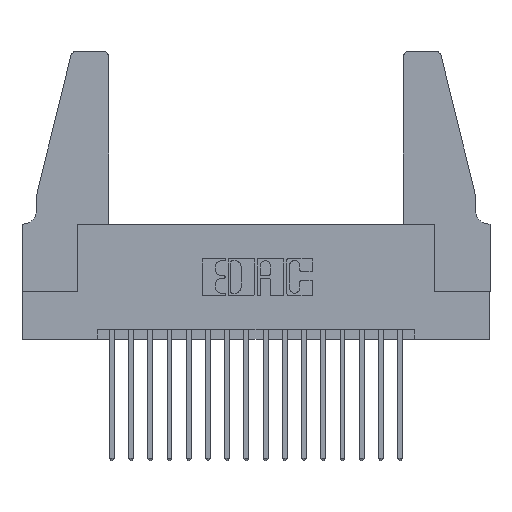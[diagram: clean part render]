
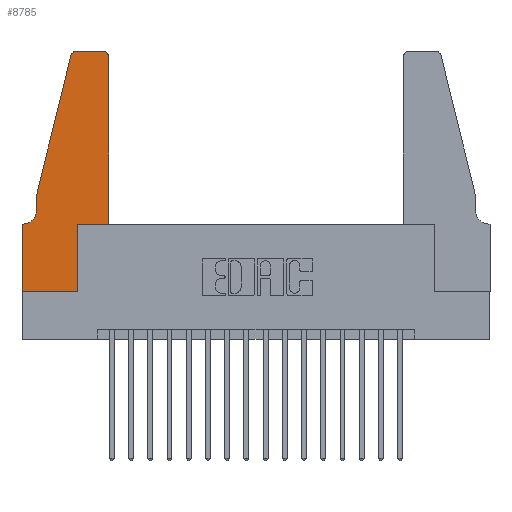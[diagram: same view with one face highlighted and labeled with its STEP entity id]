
A CAD part, top view. The second image highlights one B-rep face of the part: STEP entity #8785.
In plain terms, the highlighted planar face has unit normal (0, 0, 1).
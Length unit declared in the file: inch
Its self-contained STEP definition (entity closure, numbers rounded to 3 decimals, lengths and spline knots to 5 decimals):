
#44 = EDGE_CURVE ( 'NONE', #2629, #17191, #13344, .T. ) ;
#200 = ORIENTED_EDGE ( 'NONE', *, *, #10529, .T. ) ;
#275 = CARTESIAN_POINT ( 'NONE',  ( 0., 0., 0.37 ) ) ;
#299 = CIRCLE ( 'NONE', #2909, 0.03 ) ;
#307 = DIRECTION ( 'NONE',  ( 0., 0., 1. ) ) ;
#358 = CARTESIAN_POINT ( 'NONE',  ( 0.0755, 0.35, 0.37 ) ) ;
#796 = LINE ( 'NONE', #5725, #4197 ) ;
#1112 = VECTOR ( 'NONE', #12012, 39.37008 ) ;
#1293 = VERTEX_POINT ( 'NONE', #12576 ) ;
#1413 = ORIENTED_EDGE ( 'NONE', *, *, #2693, .T. ) ;
#1495 = ORIENTED_EDGE ( 'NONE', *, *, #4208, .T. ) ;
#1847 = EDGE_CURVE ( 'NONE', #10890, #1293, #4965, .T. ) ;
#2177 = CARTESIAN_POINT ( 'NONE',  ( 0., 0., 0.37 ) ) ;
#2473 = LINE ( 'NONE', #5337, #14990 ) ;
#2553 = ORIENTED_EDGE ( 'NONE', *, *, #11028, .T. ) ;
#2623 = EDGE_CURVE ( 'NONE', #10138, #3721, #7997, .T. ) ;
#2629 = VERTEX_POINT ( 'NONE', #18126 ) ;
#2693 = EDGE_CURVE ( 'NONE', #9091, #14931, #2473, .T. ) ;
#2798 = CIRCLE ( 'NONE', #15040, 0.03 ) ;
#2909 = AXIS2_PLACEMENT_3D ( 'NONE', #16535, #8166, #17917 ) ;
#3327 = DIRECTION ( 'NONE',  ( 0., 1., 0. ) ) ;
#3484 = CARTESIAN_POINT ( 'NONE',  ( 0.25487, 1.22718, 0.37 ) ) ;
#3504 = DIRECTION ( 'NONE',  ( -1., 0., 0. ) ) ;
#3545 = DIRECTION ( 'NONE',  ( -0.239, -0.971, 0. ) ) ;
#3574 = CARTESIAN_POINT ( 'NONE',  ( 0.2865, 0., 0.37 ) ) ;
#3633 = CARTESIAN_POINT ( 'NONE',  ( 0.2865, 0.35, 0.37 ) ) ;
#3721 = VERTEX_POINT ( 'NONE', #17758 ) ;
#4163 = CIRCLE ( 'NONE', #10090, 0.07 ) ;
#4197 = VECTOR ( 'NONE', #16907, 39.37008 ) ;
#4208 = EDGE_CURVE ( 'NONE', #12950, #10890, #7707, .T. ) ;
#4421 = EDGE_CURVE ( 'NONE', #15932, #12950, #12097, .T. ) ;
#4439 = AXIS2_PLACEMENT_3D ( 'NONE', #5583, #16766, #8406 ) ;
#4965 = LINE ( 'NONE', #11973, #1112 ) ;
#5068 = CARTESIAN_POINT ( 'NONE',  ( 0.0755, 0.5, 0.37 ) ) ;
#5165 = CARTESIAN_POINT ( 'NONE',  ( 0.0055, 0.42, 0.37 ) ) ;
#5242 = ORIENTED_EDGE ( 'NONE', *, *, #15575, .T. ) ;
#5337 = CARTESIAN_POINT ( 'NONE',  ( 0.0755, 0.5, 0.37 ) ) ;
#5452 = CARTESIAN_POINT ( 'NONE',  ( 0.2605, 1.25, 0.37 ) ) ;
#5583 = CARTESIAN_POINT ( 'NONE',  ( 0., 0.35, 0.37 ) ) ;
#5725 = CARTESIAN_POINT ( 'NONE',  ( 0.0755, 0.5, 0.37 ) ) ;
#6577 = DIRECTION ( 'NONE',  ( -1., 0., 0. ) ) ;
#6728 = LINE ( 'NONE', #8404, #17420 ) ;
#6967 = EDGE_CURVE ( 'NONE', #1293, #12687, #6728, .T. ) ;
#7138 = CARTESIAN_POINT ( 'NONE',  ( 0.4505, 1.22, 0.37 ) ) ;
#7577 = CARTESIAN_POINT ( 'NONE',  ( 0.4205, 1.25, 0.37 ) ) ;
#7707 = LINE ( 'NONE', #13160, #11421 ) ;
#7997 = LINE ( 'NONE', #5452, #14553 ) ;
#8166 = DIRECTION ( 'NONE',  ( 0., 0., 1. ) ) ;
#8404 = CARTESIAN_POINT ( 'NONE',  ( 0.4505, 0.35, 0.37 ) ) ;
#8406 = DIRECTION ( 'NONE',  ( 1., 0., 0. ) ) ;
#8519 = CARTESIAN_POINT ( 'NONE',  ( 0., 0., 0.37 ) ) ;
#8765 = EDGE_LOOP ( 'NONE', ( #14746, #9047, #1413, #200, #13914, #10304, #5242, #17519, #1495, #16688, #12825, #2553 ) ) ;
#8785 = ADVANCED_FACE ( 'NONE', ( #15851 ), #11148, .T. ) ;
#8878 = CARTESIAN_POINT ( 'NONE',  ( 0.284, 1.22, 0.37 ) ) ;
#9047 = ORIENTED_EDGE ( 'NONE', *, *, #14766, .T. ) ;
#9091 = VERTEX_POINT ( 'NONE', #3484 ) ;
#9843 = DIRECTION ( 'NONE',  ( -1., 0., 0. ) ) ;
#10039 = VECTOR ( 'NONE', #3504, 39.37008 ) ;
#10090 = AXIS2_PLACEMENT_3D ( 'NONE', #5165, #14939, #6577 ) ;
#10138 = VERTEX_POINT ( 'NONE', #7577 ) ;
#10254 = DIRECTION ( 'NONE',  ( 1., 0., 0. ) ) ;
#10304 = ORIENTED_EDGE ( 'NONE', *, *, #44, .T. ) ;
#10529 = EDGE_CURVE ( 'NONE', #14931, #17115, #796, .T. ) ;
#10890 = VERTEX_POINT ( 'NONE', #3633 ) ;
#10913 = VECTOR ( 'NONE', #15836, 39.37008 ) ;
#11028 = EDGE_CURVE ( 'NONE', #12687, #10138, #299, .T. ) ;
#11148 = PLANE ( 'NONE',  #4439 ) ;
#11421 = VECTOR ( 'NONE', #3327, 39.37008 ) ;
#11483 = EDGE_CURVE ( 'NONE', #17115, #2629, #4163, .T. ) ;
#11973 = CARTESIAN_POINT ( 'NONE',  ( 0.4505, 0.35, 0.37 ) ) ;
#12012 = DIRECTION ( 'NONE',  ( 1., 0., 0. ) ) ;
#12097 = LINE ( 'NONE', #2177, #15350 ) ;
#12100 = DIRECTION ( 'NONE',  ( 1., 0., 0. ) ) ;
#12576 = CARTESIAN_POINT ( 'NONE',  ( 0.4505, 0.35, 0.37 ) ) ;
#12687 = VERTEX_POINT ( 'NONE', #7138 ) ;
#12825 = ORIENTED_EDGE ( 'NONE', *, *, #6967, .T. ) ;
#12950 = VERTEX_POINT ( 'NONE', #3574 ) ;
#13160 = CARTESIAN_POINT ( 'NONE',  ( 0.2865, 0.35, 0.37 ) ) ;
#13344 = LINE ( 'NONE', #358, #10039 ) ;
#13682 = CARTESIAN_POINT ( 'NONE',  ( 0.0755, 0.42, 0.37 ) ) ;
#13914 = ORIENTED_EDGE ( 'NONE', *, *, #11483, .T. ) ;
#14553 = VECTOR ( 'NONE', #9843, 39.37008 ) ;
#14642 = LINE ( 'NONE', #275, #10913 ) ;
#14746 = ORIENTED_EDGE ( 'NONE', *, *, #2623, .T. ) ;
#14766 = EDGE_CURVE ( 'NONE', #3721, #9091, #2798, .T. ) ;
#14931 = VERTEX_POINT ( 'NONE', #5068 ) ;
#14939 = DIRECTION ( 'NONE',  ( 0., 0., -1. ) ) ;
#14990 = VECTOR ( 'NONE', #3545, 39.37008 ) ;
#15040 = AXIS2_PLACEMENT_3D ( 'NONE', #8878, #307, #10254 ) ;
#15240 = CARTESIAN_POINT ( 'NONE',  ( 0., 0.35, 0.37 ) ) ;
#15350 = VECTOR ( 'NONE', #12100, 39.37008 ) ;
#15575 = EDGE_CURVE ( 'NONE', #17191, #15932, #14642, .T. ) ;
#15836 = DIRECTION ( 'NONE',  ( 0., -1., 0. ) ) ;
#15851 = FACE_OUTER_BOUND ( 'NONE', #8765, .T. ) ;
#15932 = VERTEX_POINT ( 'NONE', #8519 ) ;
#16535 = CARTESIAN_POINT ( 'NONE',  ( 0.4205, 1.22, 0.37 ) ) ;
#16688 = ORIENTED_EDGE ( 'NONE', *, *, #1847, .T. ) ;
#16762 = DIRECTION ( 'NONE',  ( 0., 1., 0. ) ) ;
#16766 = DIRECTION ( 'NONE',  ( 0., 0., 1. ) ) ;
#16907 = DIRECTION ( 'NONE',  ( 0., -1., 0. ) ) ;
#17115 = VERTEX_POINT ( 'NONE', #13682 ) ;
#17191 = VERTEX_POINT ( 'NONE', #15240 ) ;
#17420 = VECTOR ( 'NONE', #16762, 39.37008 ) ;
#17519 = ORIENTED_EDGE ( 'NONE', *, *, #4421, .T. ) ;
#17758 = CARTESIAN_POINT ( 'NONE',  ( 0.284, 1.25, 0.37 ) ) ;
#17917 = DIRECTION ( 'NONE',  ( 1., 0., 0. ) ) ;
#18126 = CARTESIAN_POINT ( 'NONE',  ( 0.0055, 0.35, 0.37 ) ) ;
